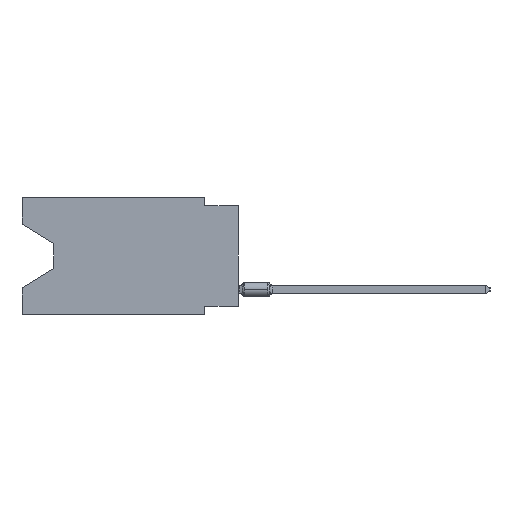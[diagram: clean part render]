
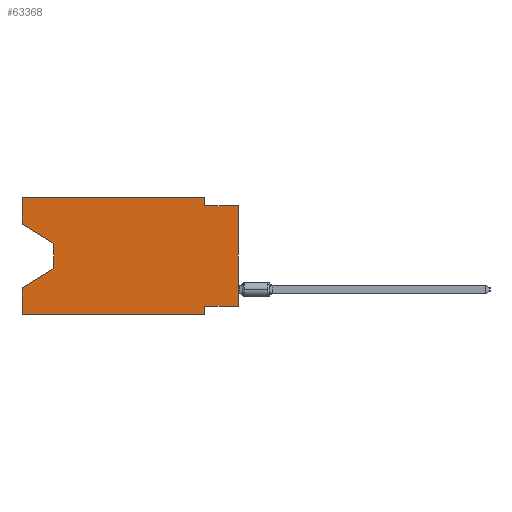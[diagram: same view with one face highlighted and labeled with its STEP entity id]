
A CAD part, left-side view. The second image highlights one B-rep face of the part: STEP entity #63368.
In plain terms, the highlighted planar face has unit normal (-1, 0, 0).
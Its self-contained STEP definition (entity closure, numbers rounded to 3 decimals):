
#1507 = EDGE_CURVE ( 'NONE', #41447, #40724, #31750, .T. ) ;
#1929 = DIRECTION ( 'NONE',  ( 0., 0., -1. ) ) ;
#4732 = EDGE_CURVE ( 'NONE', #27340, #71591, #33488, .T. ) ;
#5824 = CARTESIAN_POINT ( 'NONE',  ( 0., 16.383, -2.038 ) ) ;
#6728 = CARTESIAN_POINT ( 'NONE',  ( 0., 16.383, -2.038 ) ) ;
#7949 = LINE ( 'NONE', #64772, #55384 ) ;
#8478 = ORIENTED_EDGE ( 'NONE', *, *, #43070, .T. ) ;
#8574 = CARTESIAN_POINT ( 'NONE',  ( 0., 2.54, -8.89 ) ) ;
#9611 = ORIENTED_EDGE ( 'NONE', *, *, #12968, .T. ) ;
#9896 = VERTEX_POINT ( 'NONE', #63119 ) ;
#11046 = DIRECTION ( 'NONE',  ( 0., 0., -1. ) ) ;
#11285 = LINE ( 'NONE', #22513, #62742 ) ;
#11472 = LINE ( 'NONE', #35002, #44458 ) ;
#12630 = CARTESIAN_POINT ( 'NONE',  ( 0., 0., -8.255 ) ) ;
#12968 = EDGE_CURVE ( 'NONE', #28527, #64176, #11285, .T. ) ;
#13537 = DIRECTION ( 'NONE',  ( 0., 0., 1. ) ) ;
#16242 = ORIENTED_EDGE ( 'NONE', *, *, #50267, .F. ) ;
#16549 = DIRECTION ( 'NONE',  ( 0., -1., 0. ) ) ;
#17377 = CARTESIAN_POINT ( 'NONE',  ( 0., 0., 0. ) ) ;
#18342 = ORIENTED_EDGE ( 'NONE', *, *, #64666, .F. ) ;
#19050 = VECTOR ( 'NONE', #37369, 1000. ) ;
#20788 = CARTESIAN_POINT ( 'NONE',  ( 0., 16.383, 0. ) ) ;
#20805 = LINE ( 'NONE', #31643, #37141 ) ;
#21581 = VERTEX_POINT ( 'NONE', #12630 ) ;
#22513 = CARTESIAN_POINT ( 'NONE',  ( 0., 13.97, -5.385 ) ) ;
#22599 = CARTESIAN_POINT ( 'NONE',  ( 0., 0., -0.635 ) ) ;
#22875 = DIRECTION ( 'NONE',  ( 0., 0.855, -0.519 ) ) ;
#24339 = PLANE ( 'NONE',  #44240 ) ;
#26747 = VECTOR ( 'NONE', #16549, 1000. ) ;
#27336 = EDGE_LOOP ( 'NONE', ( #36944, #51909, #9611, #43631, #8478, #18342, #16242, #62288, #47621, #65833, #68777, #31761 ) ) ;
#27340 = VERTEX_POINT ( 'NONE', #6728 ) ;
#27666 = EDGE_CURVE ( 'NONE', #40724, #43422, #68601, .T. ) ;
#27823 = DIRECTION ( 'NONE',  ( 0., -1., 0. ) ) ;
#28467 = VERTEX_POINT ( 'NONE', #72929 ) ;
#28527 = VERTEX_POINT ( 'NONE', #46720 ) ;
#29500 = VECTOR ( 'NONE', #11046, 1000. ) ;
#30420 = LINE ( 'NONE', #48375, #49363 ) ;
#31643 = CARTESIAN_POINT ( 'NONE',  ( 0., 0., -8.255 ) ) ;
#31750 = LINE ( 'NONE', #61282, #19050 ) ;
#31761 = ORIENTED_EDGE ( 'NONE', *, *, #64129, .F. ) ;
#32471 = DIRECTION ( 'NONE',  ( 0., 0., -1. ) ) ;
#33098 = CARTESIAN_POINT ( 'NONE',  ( 0., 2.54, 0. ) ) ;
#33488 = LINE ( 'NONE', #5824, #51738 ) ;
#35002 = CARTESIAN_POINT ( 'NONE',  ( 0., 16.383, 0. ) ) ;
#36944 = ORIENTED_EDGE ( 'NONE', *, *, #4732, .T. ) ;
#37141 = VECTOR ( 'NONE', #54099, 1000. ) ;
#37369 = DIRECTION ( 'NONE',  ( 0., -1., 0. ) ) ;
#37575 = VECTOR ( 'NONE', #32471, 1000. ) ;
#38684 = LINE ( 'NONE', #22599, #49726 ) ;
#40724 = VERTEX_POINT ( 'NONE', #41468 ) ;
#41447 = VERTEX_POINT ( 'NONE', #20788 ) ;
#41468 = CARTESIAN_POINT ( 'NONE',  ( 0., 2.54, 0. ) ) ;
#42647 = EDGE_CURVE ( 'NONE', #21581, #65939, #68226, .T. ) ;
#43070 = EDGE_CURVE ( 'NONE', #28467, #61514, #44214, .T. ) ;
#43422 = VERTEX_POINT ( 'NONE', #49019 ) ;
#43631 = ORIENTED_EDGE ( 'NONE', *, *, #55795, .F. ) ;
#44214 = LINE ( 'NONE', #67044, #26747 ) ;
#44240 = AXIS2_PLACEMENT_3D ( 'NONE', #64337, #46770, #1929 ) ;
#44458 = VECTOR ( 'NONE', #69778, 1000. ) ;
#46032 = FACE_OUTER_BOUND ( 'NONE', #27336, .T. ) ;
#46720 = CARTESIAN_POINT ( 'NONE',  ( 0., 13.97, -5.385 ) ) ;
#46770 = DIRECTION ( 'NONE',  ( 1., 0., 0. ) ) ;
#47621 = ORIENTED_EDGE ( 'NONE', *, *, #59078, .F. ) ;
#48375 = CARTESIAN_POINT ( 'NONE',  ( 0., 2.54, -8.89 ) ) ;
#48599 = LINE ( 'NONE', #67253, #37575 ) ;
#49019 = CARTESIAN_POINT ( 'NONE',  ( 0., 2.54, -0.635 ) ) ;
#49363 = VECTOR ( 'NONE', #58839, 1000. ) ;
#49726 = VECTOR ( 'NONE', #27823, 1000. ) ;
#50267 = EDGE_CURVE ( 'NONE', #21581, #9896, #20805, .T. ) ;
#51738 = VECTOR ( 'NONE', #51812, 1000. ) ;
#51812 = DIRECTION ( 'NONE',  ( 0., -0.855, -0.519 ) ) ;
#51909 = ORIENTED_EDGE ( 'NONE', *, *, #56239, .T. ) ;
#54099 = DIRECTION ( 'NONE',  ( 0., 1., 0. ) ) ;
#55384 = VECTOR ( 'NONE', #13537, 1000. ) ;
#55795 = EDGE_CURVE ( 'NONE', #28467, #64176, #7949, .T. ) ;
#56239 = EDGE_CURVE ( 'NONE', #71591, #28527, #48599, .T. ) ;
#58839 = DIRECTION ( 'NONE',  ( 0., 0., -1. ) ) ;
#58869 = CARTESIAN_POINT ( 'NONE',  ( 0., 13.97, -3.505 ) ) ;
#59078 = EDGE_CURVE ( 'NONE', #43422, #65939, #38684, .T. ) ;
#61282 = CARTESIAN_POINT ( 'NONE',  ( 0., 16.383, 0. ) ) ;
#61514 = VERTEX_POINT ( 'NONE', #8574 ) ;
#62288 = ORIENTED_EDGE ( 'NONE', *, *, #42647, .T. ) ;
#62742 = VECTOR ( 'NONE', #22875, 1000. ) ;
#63119 = CARTESIAN_POINT ( 'NONE',  ( 0., 2.54, -8.255 ) ) ;
#63368 = ADVANCED_FACE ( 'NONE', ( #46032 ), #24339, .F. ) ;
#64129 = EDGE_CURVE ( 'NONE', #27340, #41447, #11472, .T. ) ;
#64176 = VERTEX_POINT ( 'NONE', #68299 ) ;
#64337 = CARTESIAN_POINT ( 'NONE',  ( 0., 16.383, 0. ) ) ;
#64666 = EDGE_CURVE ( 'NONE', #9896, #61514, #30420, .T. ) ;
#64772 = CARTESIAN_POINT ( 'NONE',  ( 0., 16.383, 0. ) ) ;
#65833 = ORIENTED_EDGE ( 'NONE', *, *, #27666, .F. ) ;
#65939 = VERTEX_POINT ( 'NONE', #68947 ) ;
#67044 = CARTESIAN_POINT ( 'NONE',  ( 0., 16.383, -8.89 ) ) ;
#67253 = CARTESIAN_POINT ( 'NONE',  ( 0., 13.97, -3.505 ) ) ;
#67860 = DIRECTION ( 'NONE',  ( 0., 0., 1. ) ) ;
#68226 = LINE ( 'NONE', #17377, #73309 ) ;
#68299 = CARTESIAN_POINT ( 'NONE',  ( 0., 16.383, -6.852 ) ) ;
#68601 = LINE ( 'NONE', #33098, #29500 ) ;
#68777 = ORIENTED_EDGE ( 'NONE', *, *, #1507, .F. ) ;
#68947 = CARTESIAN_POINT ( 'NONE',  ( 0., 0., -0.635 ) ) ;
#69778 = DIRECTION ( 'NONE',  ( 0., 0., 1. ) ) ;
#71591 = VERTEX_POINT ( 'NONE', #58869 ) ;
#72929 = CARTESIAN_POINT ( 'NONE',  ( 0., 16.383, -8.89 ) ) ;
#73309 = VECTOR ( 'NONE', #67860, 1000. ) ;
